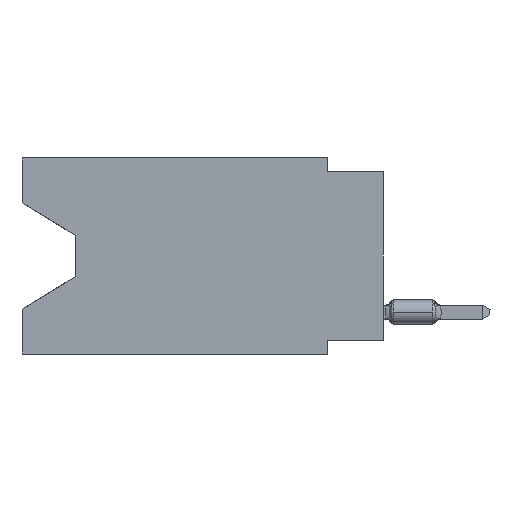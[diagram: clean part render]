
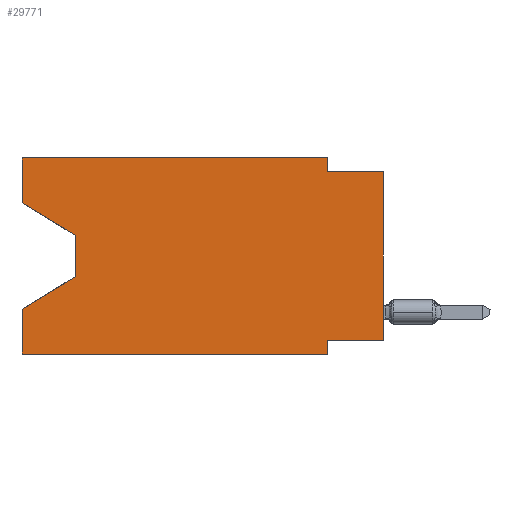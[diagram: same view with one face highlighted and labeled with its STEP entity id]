
A CAD part, left-side view. The second image highlights one B-rep face of the part: STEP entity #29771.
In plain terms, the highlighted planar face has unit normal (-1, 0, 0).
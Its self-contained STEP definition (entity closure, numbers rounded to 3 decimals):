
#401 = ORIENTED_EDGE ( 'NONE', *, *, #6923, .F. ) ;
#526 = VERTEX_POINT ( 'NONE', #4027 ) ;
#528 = CARTESIAN_POINT ( 'NONE',  ( 0., 0., -0.635 ) ) ;
#664 = CARTESIAN_POINT ( 'NONE',  ( 0., 16.383, 0. ) ) ;
#1129 = VECTOR ( 'NONE', #27617, 1000. ) ;
#1286 = LINE ( 'NONE', #10696, #20845 ) ;
#1380 = CARTESIAN_POINT ( 'NONE',  ( 0., 13.97, -3.505 ) ) ;
#2782 = CARTESIAN_POINT ( 'NONE',  ( 0., 2.54, -8.89 ) ) ;
#3446 = ORIENTED_EDGE ( 'NONE', *, *, #9088, .T. ) ;
#3575 = AXIS2_PLACEMENT_3D ( 'NONE', #664, #24728, #17175 ) ;
#3764 = CARTESIAN_POINT ( 'NONE',  ( 0., 2.54, -8.89 ) ) ;
#3783 = EDGE_CURVE ( 'NONE', #10241, #20882, #24288, .T. ) ;
#4027 = CARTESIAN_POINT ( 'NONE',  ( 0., 16.383, -8.89 ) ) ;
#4266 = LINE ( 'NONE', #14575, #16707 ) ;
#4296 = DIRECTION ( 'NONE',  ( 0., 0., -1. ) ) ;
#4417 = VECTOR ( 'NONE', #8004, 1000. ) ;
#4675 = VERTEX_POINT ( 'NONE', #21864 ) ;
#4850 = ORIENTED_EDGE ( 'NONE', *, *, #16999, .T. ) ;
#4987 = LINE ( 'NONE', #14406, #19103 ) ;
#5163 = VERTEX_POINT ( 'NONE', #15807 ) ;
#5169 = ORIENTED_EDGE ( 'NONE', *, *, #8523, .F. ) ;
#5777 = ORIENTED_EDGE ( 'NONE', *, *, #23075, .T. ) ;
#5892 = VERTEX_POINT ( 'NONE', #20528 ) ;
#5909 = EDGE_CURVE ( 'NONE', #17554, #22172, #16655, .T. ) ;
#6588 = CARTESIAN_POINT ( 'NONE',  ( 0., 2.54, 0. ) ) ;
#6662 = VECTOR ( 'NONE', #22237, 1000. ) ;
#6923 = EDGE_CURVE ( 'NONE', #526, #5892, #20677, .T. ) ;
#7366 = EDGE_CURVE ( 'NONE', #4675, #10241, #18183, .T. ) ;
#7701 = DIRECTION ( 'NONE',  ( 0., 0., -1. ) ) ;
#7788 = DIRECTION ( 'NONE',  ( 0., -1., 0. ) ) ;
#7959 = EDGE_CURVE ( 'NONE', #22172, #4675, #4987, .T. ) ;
#8004 = DIRECTION ( 'NONE',  ( 0., 1., 0. ) ) ;
#8523 = EDGE_CURVE ( 'NONE', #5163, #27442, #10325, .T. ) ;
#8635 = DIRECTION ( 'NONE',  ( 0., -0.855, -0.519 ) ) ;
#8832 = VECTOR ( 'NONE', #4296, 1000. ) ;
#8944 = CARTESIAN_POINT ( 'NONE',  ( 0., 16.383, 0. ) ) ;
#9088 = EDGE_CURVE ( 'NONE', #526, #21250, #4266, .T. ) ;
#9201 = ORIENTED_EDGE ( 'NONE', *, *, #5909, .F. ) ;
#9530 = CARTESIAN_POINT ( 'NONE',  ( 0., 13.97, -5.385 ) ) ;
#9538 = CARTESIAN_POINT ( 'NONE',  ( 0., 16.383, 0. ) ) ;
#9766 = ORIENTED_EDGE ( 'NONE', *, *, #7366, .F. ) ;
#9907 = EDGE_CURVE ( 'NONE', #17554, #23194, #14960, .T. ) ;
#9970 = CARTESIAN_POINT ( 'NONE',  ( 0., 2.54, -8.255 ) ) ;
#10001 = LINE ( 'NONE', #19413, #24679 ) ;
#10241 = VERTEX_POINT ( 'NONE', #29394 ) ;
#10325 = LINE ( 'NONE', #22355, #4417 ) ;
#10696 = CARTESIAN_POINT ( 'NONE',  ( 0., 0., 0. ) ) ;
#11814 = CARTESIAN_POINT ( 'NONE',  ( 0., 13.97, -5.385 ) ) ;
#12579 = EDGE_LOOP ( 'NONE', ( #22952, #5777, #23693, #401, #3446, #18157, #5169, #4850, #26102, #9766, #23244, #9201 ) ) ;
#14265 = DIRECTION ( 'NONE',  ( 0., -1., 0. ) ) ;
#14406 = CARTESIAN_POINT ( 'NONE',  ( 0., 16.383, 0. ) ) ;
#14575 = CARTESIAN_POINT ( 'NONE',  ( 0., 16.383, -8.89 ) ) ;
#14960 = LINE ( 'NONE', #24380, #30014 ) ;
#15807 = CARTESIAN_POINT ( 'NONE',  ( 0., 0., -8.255 ) ) ;
#16337 = DIRECTION ( 'NONE',  ( 0., 0., 1. ) ) ;
#16655 = LINE ( 'NONE', #9538, #25398 ) ;
#16707 = VECTOR ( 'NONE', #14265, 1000. ) ;
#16726 = CARTESIAN_POINT ( 'NONE',  ( 0., 16.383, 0. ) ) ;
#16999 = EDGE_CURVE ( 'NONE', #5163, #20882, #1286, .T. ) ;
#17175 = DIRECTION ( 'NONE',  ( 0., 0., -1. ) ) ;
#17554 = VERTEX_POINT ( 'NONE', #26044 ) ;
#18157 = ORIENTED_EDGE ( 'NONE', *, *, #22937, .F. ) ;
#18183 = LINE ( 'NONE', #6588, #8832 ) ;
#18601 = DIRECTION ( 'NONE',  ( 0., -1., 0. ) ) ;
#18806 = LINE ( 'NONE', #2782, #21217 ) ;
#19103 = VECTOR ( 'NONE', #18601, 1000. ) ;
#19413 = CARTESIAN_POINT ( 'NONE',  ( 0., 13.97, -3.505 ) ) ;
#20528 = CARTESIAN_POINT ( 'NONE',  ( 0., 16.383, -6.852 ) ) ;
#20677 = LINE ( 'NONE', #8944, #1129 ) ;
#20845 = VECTOR ( 'NONE', #29503, 1000. ) ;
#20882 = VERTEX_POINT ( 'NONE', #22725 ) ;
#21217 = VECTOR ( 'NONE', #25908, 1000. ) ;
#21250 = VERTEX_POINT ( 'NONE', #3764 ) ;
#21864 = CARTESIAN_POINT ( 'NONE',  ( 0., 2.54, 0. ) ) ;
#22172 = VERTEX_POINT ( 'NONE', #16726 ) ;
#22237 = DIRECTION ( 'NONE',  ( 0., 0.855, -0.519 ) ) ;
#22337 = VECTOR ( 'NONE', #7788, 1000. ) ;
#22355 = CARTESIAN_POINT ( 'NONE',  ( 0., 0., -8.255 ) ) ;
#22725 = CARTESIAN_POINT ( 'NONE',  ( 0., 0., -0.635 ) ) ;
#22937 = EDGE_CURVE ( 'NONE', #27442, #21250, #18806, .T. ) ;
#22952 = ORIENTED_EDGE ( 'NONE', *, *, #9907, .T. ) ;
#23075 = EDGE_CURVE ( 'NONE', #23194, #28867, #10001, .T. ) ;
#23194 = VERTEX_POINT ( 'NONE', #1380 ) ;
#23244 = ORIENTED_EDGE ( 'NONE', *, *, #7959, .F. ) ;
#23682 = LINE ( 'NONE', #11814, #6662 ) ;
#23693 = ORIENTED_EDGE ( 'NONE', *, *, #27821, .T. ) ;
#24288 = LINE ( 'NONE', #528, #22337 ) ;
#24380 = CARTESIAN_POINT ( 'NONE',  ( 0., 16.383, -2.038 ) ) ;
#24679 = VECTOR ( 'NONE', #7701, 1000. ) ;
#24728 = DIRECTION ( 'NONE',  ( 1., 0., 0. ) ) ;
#25398 = VECTOR ( 'NONE', #16337, 1000. ) ;
#25908 = DIRECTION ( 'NONE',  ( 0., 0., -1. ) ) ;
#26044 = CARTESIAN_POINT ( 'NONE',  ( 0., 16.383, -2.038 ) ) ;
#26102 = ORIENTED_EDGE ( 'NONE', *, *, #3783, .F. ) ;
#26727 = FACE_OUTER_BOUND ( 'NONE', #12579, .T. ) ;
#27442 = VERTEX_POINT ( 'NONE', #9970 ) ;
#27617 = DIRECTION ( 'NONE',  ( 0., 0., 1. ) ) ;
#27821 = EDGE_CURVE ( 'NONE', #28867, #5892, #23682, .T. ) ;
#28867 = VERTEX_POINT ( 'NONE', #9530 ) ;
#29052 = PLANE ( 'NONE',  #3575 ) ;
#29394 = CARTESIAN_POINT ( 'NONE',  ( 0., 2.54, -0.635 ) ) ;
#29503 = DIRECTION ( 'NONE',  ( 0., 0., 1. ) ) ;
#29771 = ADVANCED_FACE ( 'NONE', ( #26727 ), #29052, .F. ) ;
#30014 = VECTOR ( 'NONE', #8635, 1000. ) ;
